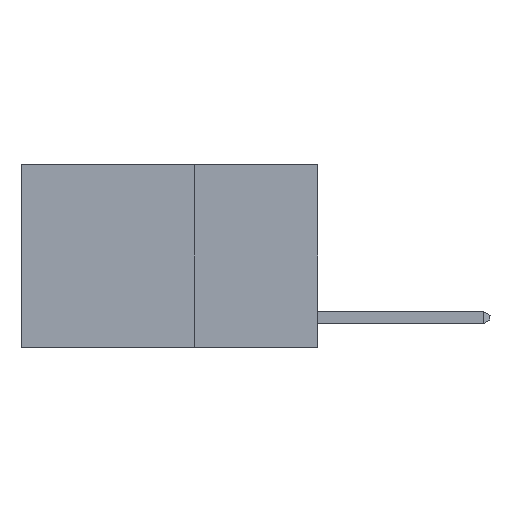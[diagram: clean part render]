
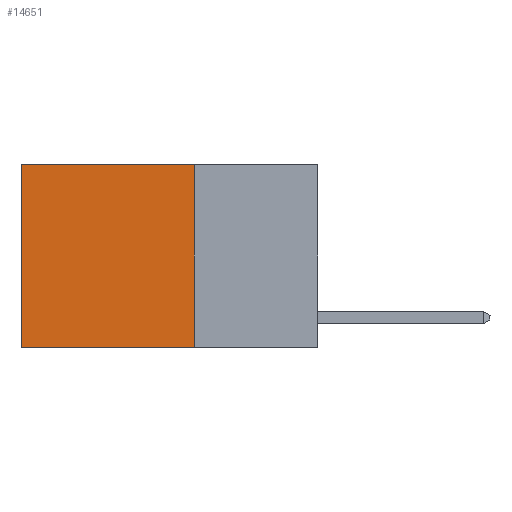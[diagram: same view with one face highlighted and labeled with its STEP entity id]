
A CAD part, left-side view. The second image highlights one B-rep face of the part: STEP entity #14651.
In plain terms, the highlighted planar face has unit normal (-1, 0, 0).
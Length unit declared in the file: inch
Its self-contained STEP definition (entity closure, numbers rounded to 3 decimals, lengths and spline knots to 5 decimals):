
#819 = CARTESIAN_POINT ( 'NONE',  ( 0.2625, 0.25, 0. ) ) ;
#3903 = EDGE_CURVE ( 'NONE', #7670, #4550, #16034, .T. ) ;
#4036 = VECTOR ( 'NONE', #6452, 39.37008 ) ;
#4550 = VERTEX_POINT ( 'NONE', #9642 ) ;
#4596 = CARTESIAN_POINT ( 'NONE',  ( 0.2625, 0.25, -0.37 ) ) ;
#4969 = DIRECTION ( 'NONE',  ( 0., 1., 0. ) ) ;
#5734 = DIRECTION ( 'NONE',  ( 1., 0., 0. ) ) ;
#6322 = CARTESIAN_POINT ( 'NONE',  ( 0.2625, 0.6, 0. ) ) ;
#6452 = DIRECTION ( 'NONE',  ( 0., 0., -1. ) ) ;
#6610 = EDGE_CURVE ( 'NONE', #7670, #7949, #15614, .T. ) ;
#7670 = VERTEX_POINT ( 'NONE', #10043 ) ;
#7949 = VERTEX_POINT ( 'NONE', #24577 ) ;
#9642 = CARTESIAN_POINT ( 'NONE',  ( 0.2625, 0.25, -0.37 ) ) ;
#10043 = CARTESIAN_POINT ( 'NONE',  ( 0.2625, 0.25, 0. ) ) ;
#10382 = ORIENTED_EDGE ( 'NONE', *, *, #16574, .T. ) ;
#10983 = ORIENTED_EDGE ( 'NONE', *, *, #3903, .F. ) ;
#11583 = ORIENTED_EDGE ( 'NONE', *, *, #6610, .T. ) ;
#11808 = CARTESIAN_POINT ( 'NONE',  ( 0.2625, 0.25, 0. ) ) ;
#13611 = VERTEX_POINT ( 'NONE', #16292 ) ;
#13724 = CARTESIAN_POINT ( 'NONE',  ( 0.2625, 0.25, 0. ) ) ;
#14100 = LINE ( 'NONE', #4596, #18349 ) ;
#14181 = LINE ( 'NONE', #6322, #4036 ) ;
#14651 = ADVANCED_FACE ( 'NONE', ( #16763 ), #24477, .F. ) ;
#15614 = LINE ( 'NONE', #13724, #17781 ) ;
#16034 = LINE ( 'NONE', #819, #16276 ) ;
#16276 = VECTOR ( 'NONE', #18074, 39.37008 ) ;
#16292 = CARTESIAN_POINT ( 'NONE',  ( 0.2625, 0.6, -0.37 ) ) ;
#16574 = EDGE_CURVE ( 'NONE', #7949, #13611, #14181, .T. ) ;
#16763 = FACE_OUTER_BOUND ( 'NONE', #22323, .T. ) ;
#17651 = DIRECTION ( 'NONE',  ( 0., 1., 0. ) ) ;
#17781 = VECTOR ( 'NONE', #17651, 39.37008 ) ;
#18074 = DIRECTION ( 'NONE',  ( 0., 0., -1. ) ) ;
#18349 = VECTOR ( 'NONE', #4969, 39.37008 ) ;
#20952 = AXIS2_PLACEMENT_3D ( 'NONE', #11808, #5734, #21197 ) ;
#21197 = DIRECTION ( 'NONE',  ( 0., 0., -1. ) ) ;
#21982 = EDGE_CURVE ( 'NONE', #4550, #13611, #14100, .T. ) ;
#22323 = EDGE_LOOP ( 'NONE', ( #10382, #24445, #10983, #11583 ) ) ;
#24445 = ORIENTED_EDGE ( 'NONE', *, *, #21982, .F. ) ;
#24477 = PLANE ( 'NONE',  #20952 ) ;
#24577 = CARTESIAN_POINT ( 'NONE',  ( 0.2625, 0.6, 0. ) ) ;
